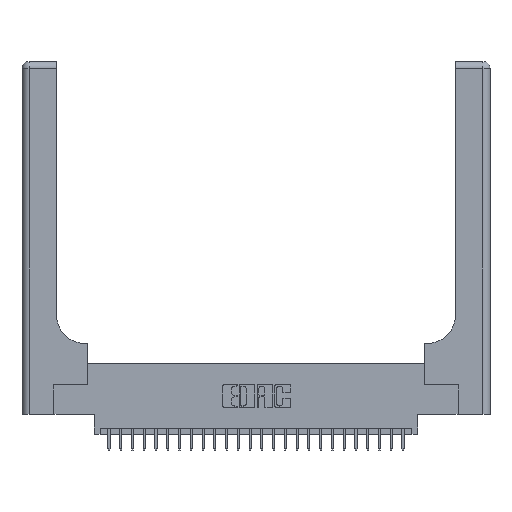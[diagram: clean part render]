
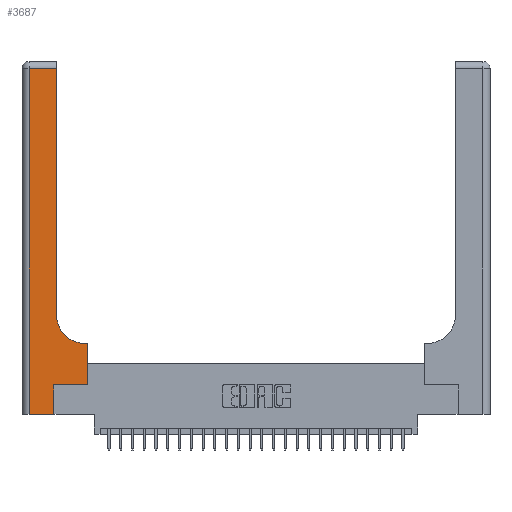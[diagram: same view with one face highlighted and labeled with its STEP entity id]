
A CAD part, top view. The second image highlights one B-rep face of the part: STEP entity #3687.
In plain terms, the highlighted planar face has unit normal (0, 0, 1).
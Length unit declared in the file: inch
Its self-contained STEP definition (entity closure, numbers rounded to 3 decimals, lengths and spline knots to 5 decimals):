
#46 = CARTESIAN_POINT ( 'NONE',  ( 0.5585, 0.6, 0.37 ) ) ;
#329 = CARTESIAN_POINT ( 'NONE',  ( 0.2915, 3., 0.37 ) ) ;
#470 = DIRECTION ( 'NONE',  ( 0., 1., 0. ) ) ;
#551 = EDGE_CURVE ( 'NONE', #25279, #22278, #6664, .T. ) ;
#836 = ORIENTED_EDGE ( 'NONE', *, *, #10689, .T. ) ;
#1173 = EDGE_CURVE ( 'NONE', #25619, #26018, #7875, .T. ) ;
#1383 = AXIS2_PLACEMENT_3D ( 'NONE', #16024, #5148, #2913 ) ;
#1527 = CARTESIAN_POINT ( 'NONE',  ( 0., 0., 0.37 ) ) ;
#1711 = PLANE ( 'NONE',  #26268 ) ;
#1766 = ORIENTED_EDGE ( 'NONE', *, *, #1173, .T. ) ;
#1853 = DIRECTION ( 'NONE',  ( 0., 0., -1. ) ) ;
#2913 = DIRECTION ( 'NONE',  ( 1., 0., 0. ) ) ;
#3687 = ADVANCED_FACE ( 'NONE', ( #21234 ), #1711, .F. ) ;
#3932 = VECTOR ( 'NONE', #11544, 39.37008 ) ;
#4957 = ORIENTED_EDGE ( 'NONE', *, *, #24622, .T. ) ;
#5148 = DIRECTION ( 'NONE',  ( 0., 0., -1. ) ) ;
#5248 = VERTEX_POINT ( 'NONE', #46 ) ;
#5334 = VERTEX_POINT ( 'NONE', #18273 ) ;
#5539 = EDGE_LOOP ( 'NONE', ( #836, #6041, #7341, #1766, #7270, #16997, #15471, #18027, #4957 ) ) ;
#5791 = VERTEX_POINT ( 'NONE', #20294 ) ;
#6041 = ORIENTED_EDGE ( 'NONE', *, *, #18269, .T. ) ;
#6664 = LINE ( 'NONE', #27754, #21626 ) ;
#6951 = CARTESIAN_POINT ( 'NONE',  ( 0.5585, 0.25, 0.37 ) ) ;
#7270 = ORIENTED_EDGE ( 'NONE', *, *, #26594, .T. ) ;
#7341 = ORIENTED_EDGE ( 'NONE', *, *, #10233, .T. ) ;
#7637 = DIRECTION ( 'NONE',  ( -1., 0., 0. ) ) ;
#7875 = LINE ( 'NONE', #1527, #13062 ) ;
#8149 = LINE ( 'NONE', #25414, #3932 ) ;
#8231 = VECTOR ( 'NONE', #10053, 39.37008 ) ;
#8661 = VECTOR ( 'NONE', #17313, 39.37008 ) ;
#9264 = CARTESIAN_POINT ( 'NONE',  ( 0.2915, 0.85, 0.37 ) ) ;
#9795 = CARTESIAN_POINT ( 'NONE',  ( 0.2915, 2.94, 0.37 ) ) ;
#9848 = CARTESIAN_POINT ( 'NONE',  ( 0.06, 0., 0.37 ) ) ;
#10053 = DIRECTION ( 'NONE',  ( 0., 1., 0. ) ) ;
#10233 = EDGE_CURVE ( 'NONE', #5791, #25619, #18333, .T. ) ;
#10689 = EDGE_CURVE ( 'NONE', #20270, #15204, #19607, .T. ) ;
#11544 = DIRECTION ( 'NONE',  ( -1., 0., 0. ) ) ;
#12562 = DIRECTION ( 'NONE',  ( 1., 0., 0. ) ) ;
#13062 = VECTOR ( 'NONE', #12562, 39.37008 ) ;
#14062 = DIRECTION ( 'NONE',  ( 0., -1., 0. ) ) ;
#14572 = CARTESIAN_POINT ( 'NONE',  ( 0.269, 0., 0.37 ) ) ;
#14714 = LINE ( 'NONE', #14572, #8231 ) ;
#15204 = VERTEX_POINT ( 'NONE', #9795 ) ;
#15471 = ORIENTED_EDGE ( 'NONE', *, *, #26234, .T. ) ;
#16024 = CARTESIAN_POINT ( 'NONE',  ( 0.5415, 0.85, 0.37 ) ) ;
#16170 = CARTESIAN_POINT ( 'NONE',  ( 0.06, 3., 0.37 ) ) ;
#16790 = CARTESIAN_POINT ( 'NONE',  ( 0., 2.94, 0.37 ) ) ;
#16997 = ORIENTED_EDGE ( 'NONE', *, *, #551, .T. ) ;
#17305 = DIRECTION ( 'NONE',  ( 1., 0., 0. ) ) ;
#17313 = DIRECTION ( 'NONE',  ( 0., 1., 0. ) ) ;
#17658 = VECTOR ( 'NONE', #470, 39.37008 ) ;
#18027 = ORIENTED_EDGE ( 'NONE', *, *, #19683, .T. ) ;
#18269 = EDGE_CURVE ( 'NONE', #15204, #5791, #25552, .T. ) ;
#18273 = CARTESIAN_POINT ( 'NONE',  ( 0.5415, 0.6, 0.37 ) ) ;
#18333 = LINE ( 'NONE', #16170, #27627 ) ;
#18959 = CARTESIAN_POINT ( 'NONE',  ( 0., 3., 0.37 ) ) ;
#19353 = CARTESIAN_POINT ( 'NONE',  ( 0.269, 0.25, 0.37 ) ) ;
#19607 = LINE ( 'NONE', #329, #17658 ) ;
#19683 = EDGE_CURVE ( 'NONE', #5248, #5334, #8149, .T. ) ;
#20270 = VERTEX_POINT ( 'NONE', #9264 ) ;
#20294 = CARTESIAN_POINT ( 'NONE',  ( 0.06, 2.94, 0.37 ) ) ;
#20379 = CIRCLE ( 'NONE', #1383, 0.25 ) ;
#20589 = CARTESIAN_POINT ( 'NONE',  ( 0.269, 0., 0.37 ) ) ;
#21234 = FACE_OUTER_BOUND ( 'NONE', #5539, .T. ) ;
#21626 = VECTOR ( 'NONE', #17305, 39.37008 ) ;
#22278 = VERTEX_POINT ( 'NONE', #22778 ) ;
#22778 = CARTESIAN_POINT ( 'NONE',  ( 0.5585, 0.25, 0.37 ) ) ;
#23944 = LINE ( 'NONE', #6951, #8661 ) ;
#24622 = EDGE_CURVE ( 'NONE', #5334, #20270, #20379, .T. ) ;
#24656 = VECTOR ( 'NONE', #25975, 39.37008 ) ;
#25279 = VERTEX_POINT ( 'NONE', #19353 ) ;
#25414 = CARTESIAN_POINT ( 'NONE',  ( 0.2915, 0.6, 0.37 ) ) ;
#25552 = LINE ( 'NONE', #16790, #24656 ) ;
#25619 = VERTEX_POINT ( 'NONE', #9848 ) ;
#25975 = DIRECTION ( 'NONE',  ( -1., 0., 0. ) ) ;
#26018 = VERTEX_POINT ( 'NONE', #20589 ) ;
#26234 = EDGE_CURVE ( 'NONE', #22278, #5248, #23944, .T. ) ;
#26268 = AXIS2_PLACEMENT_3D ( 'NONE', #18959, #1853, #7637 ) ;
#26594 = EDGE_CURVE ( 'NONE', #26018, #25279, #14714, .T. ) ;
#27627 = VECTOR ( 'NONE', #14062, 39.37008 ) ;
#27754 = CARTESIAN_POINT ( 'NONE',  ( 0.269, 0.25, 0.37 ) ) ;
